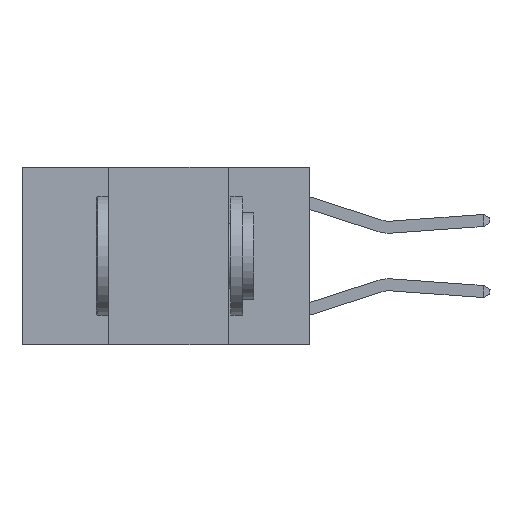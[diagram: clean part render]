
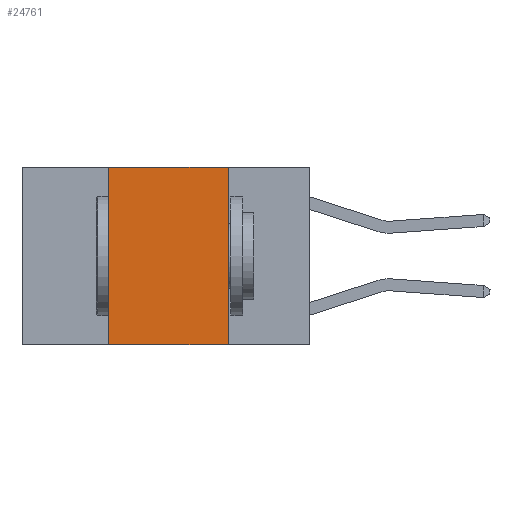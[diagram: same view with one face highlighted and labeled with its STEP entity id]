
A CAD part, left-side view. The second image highlights one B-rep face of the part: STEP entity #24761.
In plain terms, the highlighted planar face has unit normal (-1, 0, 0).
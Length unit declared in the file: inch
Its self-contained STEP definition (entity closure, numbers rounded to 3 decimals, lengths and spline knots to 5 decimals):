
#460 = VERTEX_POINT ( 'NONE', #23307 ) ;
#1845 = FACE_OUTER_BOUND ( 'NONE', #12989, .T. ) ;
#2525 = VERTEX_POINT ( 'NONE', #13145 ) ;
#3152 = CARTESIAN_POINT ( 'NONE',  ( 0., 0.17, -0.37 ) ) ;
#4940 = LINE ( 'NONE', #23466, #21311 ) ;
#5177 = EDGE_CURVE ( 'NONE', #460, #16666, #19457, .T. ) ;
#5359 = ORIENTED_EDGE ( 'NONE', *, *, #16555, .T. ) ;
#5525 = VECTOR ( 'NONE', #16870, 39.37008 ) ;
#6106 = DIRECTION ( 'NONE',  ( 0., -1., 0. ) ) ;
#6851 = AXIS2_PLACEMENT_3D ( 'NONE', #10998, #15298, #26450 ) ;
#7221 = VERTEX_POINT ( 'NONE', #3152 ) ;
#10104 = ORIENTED_EDGE ( 'NONE', *, *, #5177, .F. ) ;
#10196 = CARTESIAN_POINT ( 'NONE',  ( 0., 0.42, 0. ) ) ;
#10998 = CARTESIAN_POINT ( 'NONE',  ( 0., 0.6, 0. ) ) ;
#11421 = LINE ( 'NONE', #17814, #15930 ) ;
#11880 = EDGE_CURVE ( 'NONE', #16666, #7221, #11421, .T. ) ;
#11895 = CARTESIAN_POINT ( 'NONE',  ( 0., 0.17, 0. ) ) ;
#12989 = EDGE_LOOP ( 'NONE', ( #29180, #10104, #21636, #5359 ) ) ;
#13145 = CARTESIAN_POINT ( 'NONE',  ( 0., 0.42, -0.37 ) ) ;
#15298 = DIRECTION ( 'NONE',  ( 1., 0., 0. ) ) ;
#15930 = VECTOR ( 'NONE', #22407, 39.37008 ) ;
#16555 = EDGE_CURVE ( 'NONE', #2525, #7221, #4940, .T. ) ;
#16666 = VERTEX_POINT ( 'NONE', #11895 ) ;
#16870 = DIRECTION ( 'NONE',  ( 0., 0., 1. ) ) ;
#16911 = CARTESIAN_POINT ( 'NONE',  ( 0., 0.6, 0. ) ) ;
#17814 = CARTESIAN_POINT ( 'NONE',  ( 0., 0.17, 0. ) ) ;
#19457 = LINE ( 'NONE', #16911, #21670 ) ;
#20075 = PLANE ( 'NONE',  #6851 ) ;
#21268 = DIRECTION ( 'NONE',  ( 0., -1., 0. ) ) ;
#21311 = VECTOR ( 'NONE', #21268, 39.37008 ) ;
#21636 = ORIENTED_EDGE ( 'NONE', *, *, #26935, .F. ) ;
#21670 = VECTOR ( 'NONE', #6106, 39.37008 ) ;
#22407 = DIRECTION ( 'NONE',  ( 0., 0., -1. ) ) ;
#23307 = CARTESIAN_POINT ( 'NONE',  ( 0., 0.42, 0. ) ) ;
#23466 = CARTESIAN_POINT ( 'NONE',  ( 0., 0.6, -0.37 ) ) ;
#24761 = ADVANCED_FACE ( 'NONE', ( #1845 ), #20075, .F. ) ;
#25339 = LINE ( 'NONE', #10196, #5525 ) ;
#26450 = DIRECTION ( 'NONE',  ( 0., 0., -1. ) ) ;
#26935 = EDGE_CURVE ( 'NONE', #2525, #460, #25339, .T. ) ;
#29180 = ORIENTED_EDGE ( 'NONE', *, *, #11880, .F. ) ;
